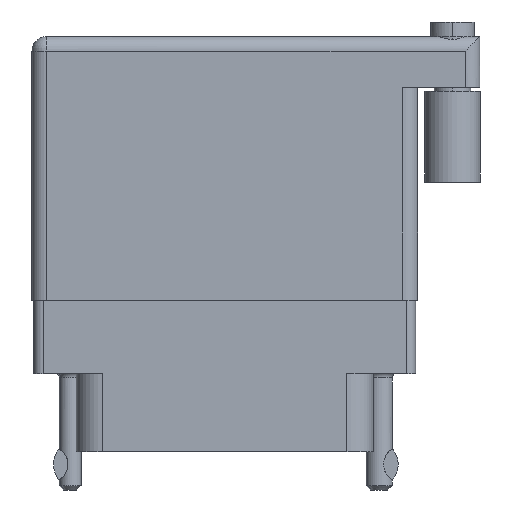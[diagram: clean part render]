
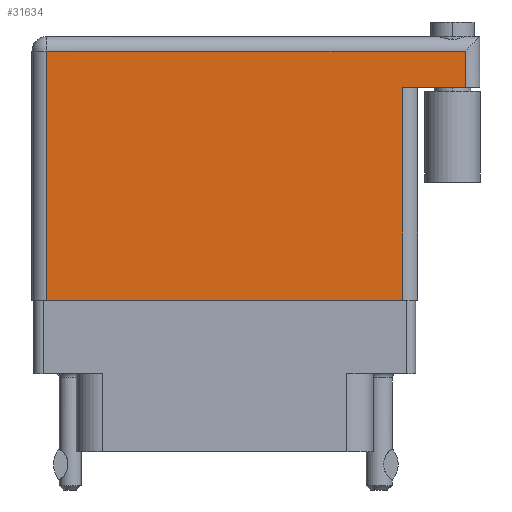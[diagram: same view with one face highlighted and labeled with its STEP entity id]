
A CAD part, front view. The second image highlights one B-rep face of the part: STEP entity #31634.
In plain terms, the highlighted face is planar.
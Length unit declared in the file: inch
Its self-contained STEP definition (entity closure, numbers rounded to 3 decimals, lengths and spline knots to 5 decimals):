
#177 = EDGE_CURVE ( 'NONE', #10773, #10016, #35556, .T. ) ;
#250 = VECTOR ( 'NONE', #12700, 39.37008 ) ;
#552 = FACE_OUTER_BOUND ( 'NONE', #26597, .T. ) ;
#3997 = DIRECTION ( 'NONE',  ( 1., 0., 0. ) ) ;
#4250 = EDGE_CURVE ( 'NONE', #10016, #17904, #22147, .T. ) ;
#4751 = DIRECTION ( 'NONE',  ( -1., 0., 0. ) ) ;
#6187 = VECTOR ( 'NONE', #19011, 39.37008 ) ;
#6219 = ORIENTED_EDGE ( 'NONE', *, *, #16598, .T. ) ;
#6902 = CARTESIAN_POINT ( 'NONE',  ( 1.539, 0.731, 0. ) ) ;
#7101 = VERTEX_POINT ( 'NONE', #19736 ) ;
#9026 = EDGE_CURVE ( 'NONE', #25319, #7101, #25395, .T. ) ;
#9881 = CARTESIAN_POINT ( 'NONE',  ( 1.489, 0.906, 0. ) ) ;
#10016 = VERTEX_POINT ( 'NONE', #25793 ) ;
#10152 = CARTESIAN_POINT ( 'NONE',  ( 0., 0.856, 0. ) ) ;
#10773 = VERTEX_POINT ( 'NONE', #12500 ) ;
#10980 = VECTOR ( 'NONE', #16870, 39.37008 ) ;
#10999 = CARTESIAN_POINT ( 'NONE',  ( 0.05, 0., 0. ) ) ;
#11391 = CARTESIAN_POINT ( 'NONE',  ( 0.05, 0., 0. ) ) ;
#11636 = EDGE_CURVE ( 'NONE', #22420, #7101, #33513, .T. ) ;
#12335 = ORIENTED_EDGE ( 'NONE', *, *, #18595, .T. ) ;
#12500 = CARTESIAN_POINT ( 'NONE',  ( 1.489, 0.856, 0. ) ) ;
#12700 = DIRECTION ( 'NONE',  ( -1., 0., 0. ) ) ;
#13423 = CARTESIAN_POINT ( 'NONE',  ( 1.489, 0.731, 0. ) ) ;
#15624 = CARTESIAN_POINT ( 'NONE',  ( 1.275, 0., 0. ) ) ;
#16598 = EDGE_CURVE ( 'NONE', #22420, #10773, #24150, .T. ) ;
#16870 = DIRECTION ( 'NONE',  ( 0., -1., 0. ) ) ;
#17904 = VERTEX_POINT ( 'NONE', #10999 ) ;
#18595 = EDGE_CURVE ( 'NONE', #17904, #25319, #33964, .T. ) ;
#19011 = DIRECTION ( 'NONE',  ( -1., 0., 0. ) ) ;
#19736 = CARTESIAN_POINT ( 'NONE',  ( 1.275, 0.731, 0. ) ) ;
#20856 = CARTESIAN_POINT ( 'NONE',  ( 0., 0., 0. ) ) ;
#21476 = CARTESIAN_POINT ( 'NONE',  ( 0., 0.906, 0. ) ) ;
#21906 = VECTOR ( 'NONE', #3997, 39.37008 ) ;
#22102 = DIRECTION ( 'NONE',  ( 0., 1., 0. ) ) ;
#22147 = LINE ( 'NONE', #11391, #10980 ) ;
#22420 = VERTEX_POINT ( 'NONE', #13423 ) ;
#22965 = ORIENTED_EDGE ( 'NONE', *, *, #9026, .T. ) ;
#23266 = VECTOR ( 'NONE', #26376, 39.37008 ) ;
#23511 = ORIENTED_EDGE ( 'NONE', *, *, #11636, .F. ) ;
#23901 = PLANE ( 'NONE',  #24276 ) ;
#24150 = LINE ( 'NONE', #9881, #23266 ) ;
#24276 = AXIS2_PLACEMENT_3D ( 'NONE', #21476, #26672, #4751 ) ;
#25319 = VERTEX_POINT ( 'NONE', #15624 ) ;
#25395 = LINE ( 'NONE', #27672, #34021 ) ;
#25793 = CARTESIAN_POINT ( 'NONE',  ( 0.05, 0.856, 0. ) ) ;
#26376 = DIRECTION ( 'NONE',  ( 0., 1., 0. ) ) ;
#26597 = EDGE_LOOP ( 'NONE', ( #12335, #22965, #23511, #6219, #31365, #31036 ) ) ;
#26672 = DIRECTION ( 'NONE',  ( 0., 0., -1. ) ) ;
#27672 = CARTESIAN_POINT ( 'NONE',  ( 1.275, 0.731, 0. ) ) ;
#31036 = ORIENTED_EDGE ( 'NONE', *, *, #4250, .T. ) ;
#31365 = ORIENTED_EDGE ( 'NONE', *, *, #177, .T. ) ;
#31634 = ADVANCED_FACE ( 'NONE', ( #552 ), #23901, .F. ) ;
#33513 = LINE ( 'NONE', #6902, #250 ) ;
#33964 = LINE ( 'NONE', #20856, #21906 ) ;
#34021 = VECTOR ( 'NONE', #22102, 39.37008 ) ;
#35556 = LINE ( 'NONE', #10152, #6187 ) ;
